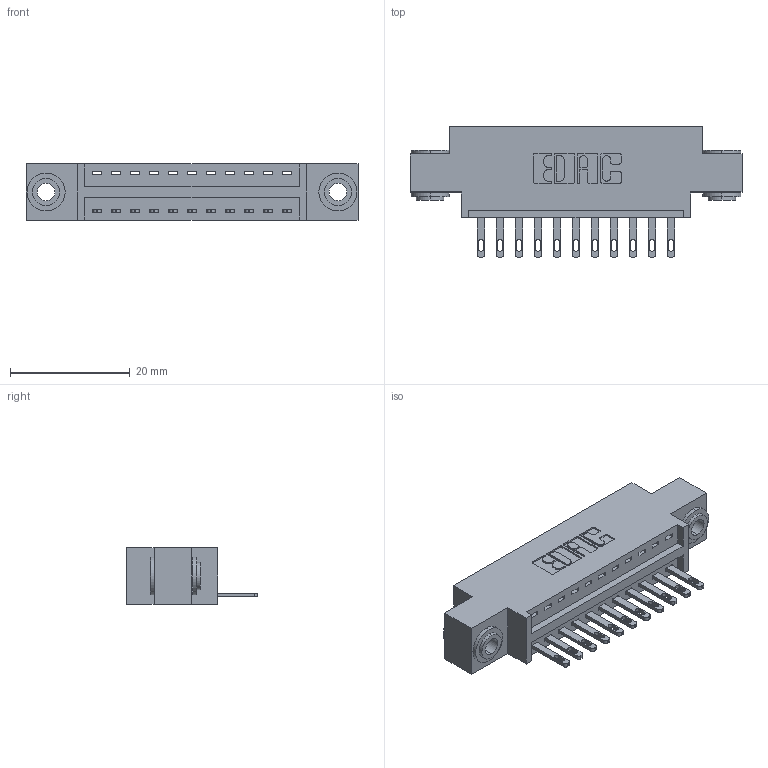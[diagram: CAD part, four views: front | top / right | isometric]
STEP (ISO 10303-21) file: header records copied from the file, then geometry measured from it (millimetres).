
FILE_DESCRIPTION (( 'STEP AP203' ), '1' );
FILE_NAME ('896-011-500-603.STEP', '2021-07-27T14:36:30', ( '' ), ( '' ), 'SwSTEP 2.0', 'SolidWorks 2020', '' );
FILE_SCHEMA (( 'CONFIG_CONTROL_DESIGN' ));
Length unit declared in the file: inch
Products named in the file (4): 896-011-500-603; 846 Part_0.170 Offset - 0.156 Dia-TH; 345-250-002_345-250-002-102; 345-292-001_345-293-100
Assembly tree (14 placements, depth 2):
  896-011-500-603
    846 Part_0.170 Offset - 0.156 Dia-TH
    345-292-001_345-293-100  x11
    345-250-002_345-250-002-102  x2
Bounding box: 55.5 x 21.84 x 9.4 mm (x, y, z)
Volume: 4970.5 mm3; surface area: 6283.1 mm2
Topology: 14 solids, 14 shells, 758 faces, 2265 edges, 1506 vertices
Faces by surface type: plane 464, cylinder 286, cone 8
Entity records: 11712 total; most frequent: CARTESIAN_POINT 1996, ORIENTED_EDGE 1934, DIRECTION 1831, EDGE_CURVE 967, LINE 763, VECTOR 763, VERTEX_POINT 642, AXIS2_PLACEMENT_3D 534
